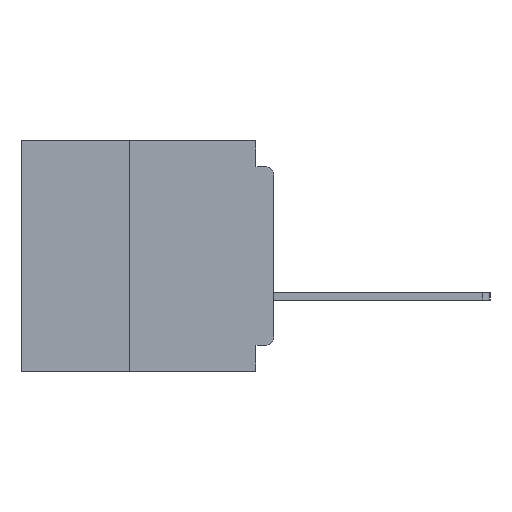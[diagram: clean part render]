
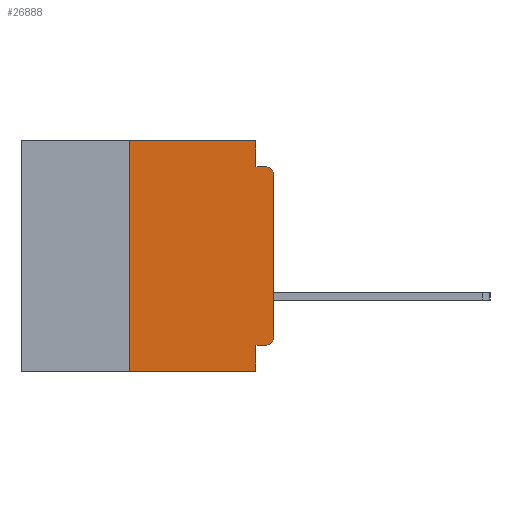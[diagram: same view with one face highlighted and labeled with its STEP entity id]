
A CAD part, left-side view. The second image highlights one B-rep face of the part: STEP entity #26888.
In plain terms, the highlighted planar face has unit normal (-1, 0, 0).
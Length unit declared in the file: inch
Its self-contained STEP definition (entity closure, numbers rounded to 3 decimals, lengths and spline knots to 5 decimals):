
#1251 = EDGE_CURVE ( 'NONE', #30298, #23978, #42760, .T. ) ;
#1403 = EDGE_CURVE ( 'NONE', #50107, #7801, #2360, .T. ) ;
#1603 = VERTEX_POINT ( 'NONE', #30344 ) ;
#2360 = CIRCLE ( 'NONE', #26372, 0.015 ) ;
#2642 = CARTESIAN_POINT ( 'NONE',  ( 0., 0.031, 0. ) ) ;
#3157 = EDGE_LOOP ( 'NONE', ( #19698, #38839, #17565, #51974, #3899, #49010, #30761, #14570, #13130, #29594 ) ) ;
#3316 = CARTESIAN_POINT ( 'NONE',  ( 0., 0.015, -0.06 ) ) ;
#3358 = VECTOR ( 'NONE', #31304, 39.37008 ) ;
#3674 = LINE ( 'NONE', #50677, #24843 ) ;
#3899 = ORIENTED_EDGE ( 'NONE', *, *, #32496, .F. ) ;
#4275 = VECTOR ( 'NONE', #34318, 39.37008 ) ;
#4750 = CARTESIAN_POINT ( 'NONE',  ( 0., 0.031, -0.4 ) ) ;
#7598 = DIRECTION ( 'NONE',  ( 0., 0., -1. ) ) ;
#7801 = VERTEX_POINT ( 'NONE', #32785 ) ;
#7822 = EDGE_CURVE ( 'NONE', #53391, #31428, #44121, .T. ) ;
#7991 = EDGE_CURVE ( 'NONE', #33703, #33762, #3674, .T. ) ;
#8945 = CARTESIAN_POINT ( 'NONE',  ( 0., 0.437, 0. ) ) ;
#10749 = AXIS2_PLACEMENT_3D ( 'NONE', #8945, #30049, #17444 ) ;
#12680 = CARTESIAN_POINT ( 'NONE',  ( 0., 0.437, 0. ) ) ;
#12958 = CARTESIAN_POINT ( 'NONE',  ( 0., 0., -0.06 ) ) ;
#13130 = ORIENTED_EDGE ( 'NONE', *, *, #35162, .F. ) ;
#13215 = PLANE ( 'NONE',  #10749 ) ;
#14244 = EDGE_CURVE ( 'NONE', #23978, #31428, #22271, .T. ) ;
#14431 = CARTESIAN_POINT ( 'NONE',  ( 0., 0., -0.355 ) ) ;
#14529 = LINE ( 'NONE', #15648, #46966 ) ;
#14570 = ORIENTED_EDGE ( 'NONE', *, *, #7991, .F. ) ;
#14574 = CARTESIAN_POINT ( 'NONE',  ( 0., 0.25, 0. ) ) ;
#14658 = LINE ( 'NONE', #39785, #3358 ) ;
#15588 = VECTOR ( 'NONE', #20999, 39.37008 ) ;
#15648 = CARTESIAN_POINT ( 'NONE',  ( 0., 0.437, -0.4 ) ) ;
#16494 = EDGE_CURVE ( 'NONE', #1603, #33762, #14529, .T. ) ;
#17444 = DIRECTION ( 'NONE',  ( 0., 0., -1. ) ) ;
#17565 = ORIENTED_EDGE ( 'NONE', *, *, #14244, .F. ) ;
#18223 = LINE ( 'NONE', #12680, #15588 ) ;
#19698 = ORIENTED_EDGE ( 'NONE', *, *, #45436, .T. ) ;
#19899 = DIRECTION ( 'NONE',  ( 0., -1., 0. ) ) ;
#20233 = VECTOR ( 'NONE', #45000, 39.37008 ) ;
#20542 = VECTOR ( 'NONE', #27148, 39.37008 ) ;
#20999 = DIRECTION ( 'NONE',  ( 0., -1., 0. ) ) ;
#21289 = VERTEX_POINT ( 'NONE', #14574 ) ;
#22271 = LINE ( 'NONE', #41992, #54663 ) ;
#23978 = VERTEX_POINT ( 'NONE', #44914 ) ;
#24843 = VECTOR ( 'NONE', #29598, 39.37008 ) ;
#26372 = AXIS2_PLACEMENT_3D ( 'NONE', #37332, #37263, #37148 ) ;
#26888 = ADVANCED_FACE ( 'NONE', ( #39538 ), #13215, .F. ) ;
#27148 = DIRECTION ( 'NONE',  ( 0., 1., 0. ) ) ;
#29010 = DIRECTION ( 'NONE',  ( 0., -1., 0. ) ) ;
#29594 = ORIENTED_EDGE ( 'NONE', *, *, #1403, .T. ) ;
#29598 = DIRECTION ( 'NONE',  ( 0., 0., -1. ) ) ;
#30019 = CARTESIAN_POINT ( 'NONE',  ( 0., 0., 0. ) ) ;
#30049 = DIRECTION ( 'NONE',  ( 1., 0., 0. ) ) ;
#30298 = VERTEX_POINT ( 'NONE', #2642 ) ;
#30344 = CARTESIAN_POINT ( 'NONE',  ( 0., 0.25, -0.4 ) ) ;
#30761 = ORIENTED_EDGE ( 'NONE', *, *, #16494, .T. ) ;
#31304 = DIRECTION ( 'NONE',  ( 0., 0., 1. ) ) ;
#31428 = VERTEX_POINT ( 'NONE', #42570 ) ;
#32292 = CARTESIAN_POINT ( 'NONE',  ( 0., 0.015, -0.355 ) ) ;
#32496 = EDGE_CURVE ( 'NONE', #21289, #30298, #18223, .T. ) ;
#32785 = CARTESIAN_POINT ( 'NONE',  ( 0., 0., -0.34 ) ) ;
#32968 = DIRECTION ( 'NONE',  ( -1., 0., 0. ) ) ;
#33703 = VERTEX_POINT ( 'NONE', #50819 ) ;
#33762 = VERTEX_POINT ( 'NONE', #4750 ) ;
#34318 = DIRECTION ( 'NONE',  ( 0., 0., 1. ) ) ;
#35162 = EDGE_CURVE ( 'NONE', #50107, #33703, #43072, .T. ) ;
#37148 = DIRECTION ( 'NONE',  ( 0., 0., -1. ) ) ;
#37263 = DIRECTION ( 'NONE',  ( -1., 0., 0. ) ) ;
#37332 = CARTESIAN_POINT ( 'NONE',  ( 0., 0.015, -0.34 ) ) ;
#38062 = LINE ( 'NONE', #30019, #4275 ) ;
#38839 = ORIENTED_EDGE ( 'NONE', *, *, #7822, .T. ) ;
#39538 = FACE_OUTER_BOUND ( 'NONE', #3157, .T. ) ;
#39785 = CARTESIAN_POINT ( 'NONE',  ( 0., 0.25, -0.4 ) ) ;
#41992 = CARTESIAN_POINT ( 'NONE',  ( 0., 0., -0.045 ) ) ;
#42052 = EDGE_CURVE ( 'NONE', #1603, #21289, #14658, .T. ) ;
#42570 = CARTESIAN_POINT ( 'NONE',  ( 0., 0.015, -0.045 ) ) ;
#42760 = LINE ( 'NONE', #45902, #20233 ) ;
#43072 = LINE ( 'NONE', #14431, #20542 ) ;
#44121 = CIRCLE ( 'NONE', #47988, 0.015 ) ;
#44914 = CARTESIAN_POINT ( 'NONE',  ( 0., 0.031, -0.045 ) ) ;
#45000 = DIRECTION ( 'NONE',  ( 0., 0., -1. ) ) ;
#45436 = EDGE_CURVE ( 'NONE', #7801, #53391, #38062, .T. ) ;
#45902 = CARTESIAN_POINT ( 'NONE',  ( 0., 0.031, 0. ) ) ;
#46966 = VECTOR ( 'NONE', #19899, 39.37008 ) ;
#47988 = AXIS2_PLACEMENT_3D ( 'NONE', #3316, #32968, #7598 ) ;
#49010 = ORIENTED_EDGE ( 'NONE', *, *, #42052, .F. ) ;
#50107 = VERTEX_POINT ( 'NONE', #32292 ) ;
#50677 = CARTESIAN_POINT ( 'NONE',  ( 0., 0.031, -0.4 ) ) ;
#50819 = CARTESIAN_POINT ( 'NONE',  ( 0., 0.031, -0.355 ) ) ;
#51974 = ORIENTED_EDGE ( 'NONE', *, *, #1251, .F. ) ;
#53391 = VERTEX_POINT ( 'NONE', #12958 ) ;
#54663 = VECTOR ( 'NONE', #29010, 39.37008 ) ;
